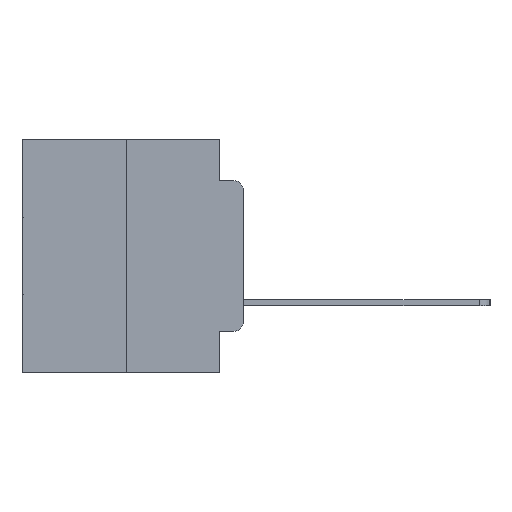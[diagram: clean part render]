
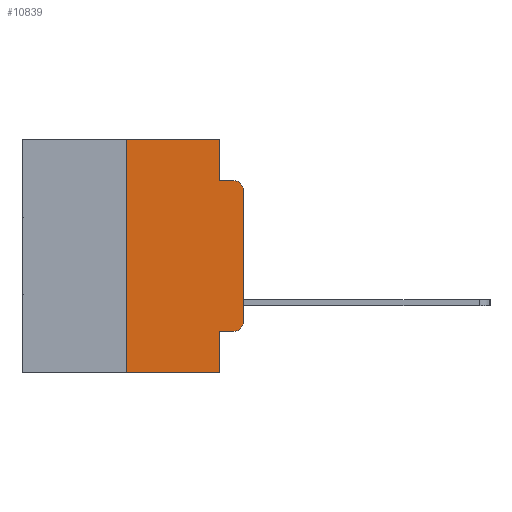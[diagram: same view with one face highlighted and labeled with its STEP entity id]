
A CAD part, left-side view. The second image highlights one B-rep face of the part: STEP entity #10839.
In plain terms, the highlighted planar face has unit normal (-1, 0, 0).
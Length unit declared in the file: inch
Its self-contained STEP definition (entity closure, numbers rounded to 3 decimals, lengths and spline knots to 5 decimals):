
#711 = ORIENTED_EDGE ( 'NONE', *, *, #13233, .F. ) ;
#913 = CARTESIAN_POINT ( 'NONE',  ( 0., 0.051, 0. ) ) ;
#1098 = ORIENTED_EDGE ( 'NONE', *, *, #6616, .T. ) ;
#1285 = VECTOR ( 'NONE', #15742, 39.37008 ) ;
#1300 = VERTEX_POINT ( 'NONE', #9537 ) ;
#1860 = ORIENTED_EDGE ( 'NONE', *, *, #16647, .T. ) ;
#1963 = VERTEX_POINT ( 'NONE', #11855 ) ;
#1992 = ORIENTED_EDGE ( 'NONE', *, *, #12263, .T. ) ;
#2007 = LINE ( 'NONE', #16122, #19371 ) ;
#2645 = ORIENTED_EDGE ( 'NONE', *, *, #20369, .T. ) ;
#2653 = ORIENTED_EDGE ( 'NONE', *, *, #21931, .F. ) ;
#2946 = CARTESIAN_POINT ( 'NONE',  ( 0., 0.473, 0. ) ) ;
#2969 = VERTEX_POINT ( 'NONE', #8307 ) ;
#3211 = LINE ( 'NONE', #17531, #21244 ) ;
#3217 = DIRECTION ( 'NONE',  ( 1., 0., 0. ) ) ;
#3534 = EDGE_CURVE ( 'NONE', #5524, #23080, #16633, .T. ) ;
#3978 = DIRECTION ( 'NONE',  ( 0., -1., 0. ) ) ;
#4171 = CARTESIAN_POINT ( 'NONE',  ( 0., 0.051, -0.5 ) ) ;
#4455 = CARTESIAN_POINT ( 'NONE',  ( 0., 0.473, -0.5 ) ) ;
#4583 = CARTESIAN_POINT ( 'NONE',  ( 0., 0.02, -0.4115 ) ) ;
#4821 = DIRECTION ( 'NONE',  ( 0., 0., 1. ) ) ;
#4897 = CARTESIAN_POINT ( 'NONE',  ( 0., 0.25, -0.5 ) ) ;
#5037 = DIRECTION ( 'NONE',  ( -1., 0., 0. ) ) ;
#5098 = VERTEX_POINT ( 'NONE', #16207 ) ;
#5463 = CARTESIAN_POINT ( 'NONE',  ( 0., 0.473, 0. ) ) ;
#5524 = VERTEX_POINT ( 'NONE', #25160 ) ;
#5715 = CARTESIAN_POINT ( 'NONE',  ( 0., 0.02, -0.0885 ) ) ;
#6616 = EDGE_CURVE ( 'NONE', #1300, #1963, #18933, .T. ) ;
#6969 = VECTOR ( 'NONE', #4821, 39.37008 ) ;
#7161 = CIRCLE ( 'NONE', #20325, 0.02 ) ;
#7590 = EDGE_LOOP ( 'NONE', ( #1098, #1860, #15184, #13386, #10438, #2653, #1992, #711, #2645, #8643 ) ) ;
#8307 = CARTESIAN_POINT ( 'NONE',  ( 0., 0.051, -0.4115 ) ) ;
#8643 = ORIENTED_EDGE ( 'NONE', *, *, #21859, .T. ) ;
#9405 = CARTESIAN_POINT ( 'NONE',  ( 0., 0., 0. ) ) ;
#9537 = CARTESIAN_POINT ( 'NONE',  ( 0., 0., -0.3915 ) ) ;
#9942 = VECTOR ( 'NONE', #13997, 39.37008 ) ;
#10082 = DIRECTION ( 'NONE',  ( 0., 0., -1. ) ) ;
#10438 = ORIENTED_EDGE ( 'NONE', *, *, #28463, .F. ) ;
#10839 = ADVANCED_FACE ( 'NONE', ( #24231 ), #16802, .F. ) ;
#10966 = CARTESIAN_POINT ( 'NONE',  ( 0., 0.051, -0.0885 ) ) ;
#11384 = CARTESIAN_POINT ( 'NONE',  ( 0., 0.02, -0.3915 ) ) ;
#11663 = VERTEX_POINT ( 'NONE', #4171 ) ;
#11741 = VECTOR ( 'NONE', #18780, 39.37008 ) ;
#11855 = CARTESIAN_POINT ( 'NONE',  ( 0., 0., -0.1085 ) ) ;
#12263 = EDGE_CURVE ( 'NONE', #26166, #11663, #19387, .T. ) ;
#13233 = EDGE_CURVE ( 'NONE', #2969, #11663, #17941, .T. ) ;
#13363 = VECTOR ( 'NONE', #10082, 39.37008 ) ;
#13386 = ORIENTED_EDGE ( 'NONE', *, *, #3534, .F. ) ;
#13669 = DIRECTION ( 'NONE',  ( 0., 0., -1. ) ) ;
#13997 = DIRECTION ( 'NONE',  ( 0., 0., -1. ) ) ;
#14173 = CARTESIAN_POINT ( 'NONE',  ( 0., 0.051, 0. ) ) ;
#14205 = CARTESIAN_POINT ( 'NONE',  ( 0., 0.051, -0.0885 ) ) ;
#15184 = ORIENTED_EDGE ( 'NONE', *, *, #18321, .F. ) ;
#15742 = DIRECTION ( 'NONE',  ( 0., -1., 0. ) ) ;
#16067 = VECTOR ( 'NONE', #17669, 39.37008 ) ;
#16122 = CARTESIAN_POINT ( 'NONE',  ( 0., 0.25, 0. ) ) ;
#16207 = CARTESIAN_POINT ( 'NONE',  ( 0., 0.25, 0. ) ) ;
#16633 = LINE ( 'NONE', #14173, #9942 ) ;
#16647 = EDGE_CURVE ( 'NONE', #1963, #20251, #7161, .T. ) ;
#16778 = LINE ( 'NONE', #10966, #16067 ) ;
#16802 = PLANE ( 'NONE',  #23927 ) ;
#17175 = VERTEX_POINT ( 'NONE', #4583 ) ;
#17531 = CARTESIAN_POINT ( 'NONE',  ( 0., 0.051, -0.4115 ) ) ;
#17669 = DIRECTION ( 'NONE',  ( 0., -1., 0. ) ) ;
#17730 = LINE ( 'NONE', #2946, #11741 ) ;
#17941 = LINE ( 'NONE', #913, #13363 ) ;
#18321 = EDGE_CURVE ( 'NONE', #23080, #20251, #16778, .T. ) ;
#18380 = DIRECTION ( 'NONE',  ( 0., 0., 1. ) ) ;
#18546 = CARTESIAN_POINT ( 'NONE',  ( 0., 0.02, -0.1085 ) ) ;
#18780 = DIRECTION ( 'NONE',  ( 0., -1., 0. ) ) ;
#18933 = LINE ( 'NONE', #9405, #6969 ) ;
#19032 = DIRECTION ( 'NONE',  ( 0., 0., -1. ) ) ;
#19371 = VECTOR ( 'NONE', #18380, 39.37008 ) ;
#19387 = LINE ( 'NONE', #4455, #1285 ) ;
#20251 = VERTEX_POINT ( 'NONE', #5715 ) ;
#20325 = AXIS2_PLACEMENT_3D ( 'NONE', #18546, #5037, #20790 ) ;
#20369 = EDGE_CURVE ( 'NONE', #2969, #17175, #3211, .T. ) ;
#20790 = DIRECTION ( 'NONE',  ( 0., 0., -1. ) ) ;
#21244 = VECTOR ( 'NONE', #3978, 39.37008 ) ;
#21859 = EDGE_CURVE ( 'NONE', #17175, #1300, #27962, .T. ) ;
#21931 = EDGE_CURVE ( 'NONE', #26166, #5098, #2007, .T. ) ;
#23080 = VERTEX_POINT ( 'NONE', #14205 ) ;
#23759 = AXIS2_PLACEMENT_3D ( 'NONE', #11384, #26944, #13669 ) ;
#23927 = AXIS2_PLACEMENT_3D ( 'NONE', #5463, #3217, #19032 ) ;
#24231 = FACE_OUTER_BOUND ( 'NONE', #7590, .T. ) ;
#25160 = CARTESIAN_POINT ( 'NONE',  ( 0., 0.051, 0. ) ) ;
#26166 = VERTEX_POINT ( 'NONE', #4897 ) ;
#26944 = DIRECTION ( 'NONE',  ( -1., 0., 0. ) ) ;
#27962 = CIRCLE ( 'NONE', #23759, 0.02 ) ;
#28463 = EDGE_CURVE ( 'NONE', #5098, #5524, #17730, .T. ) ;
